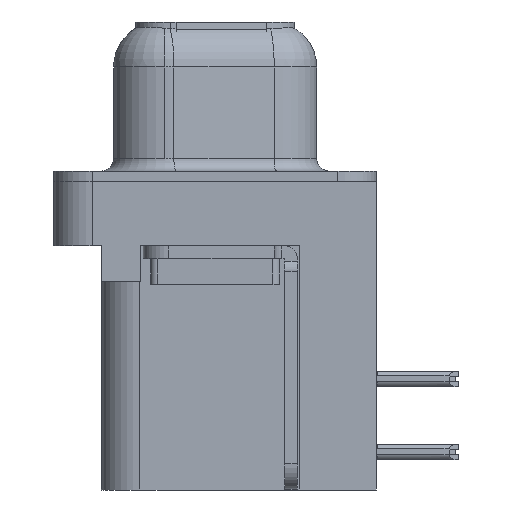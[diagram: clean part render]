
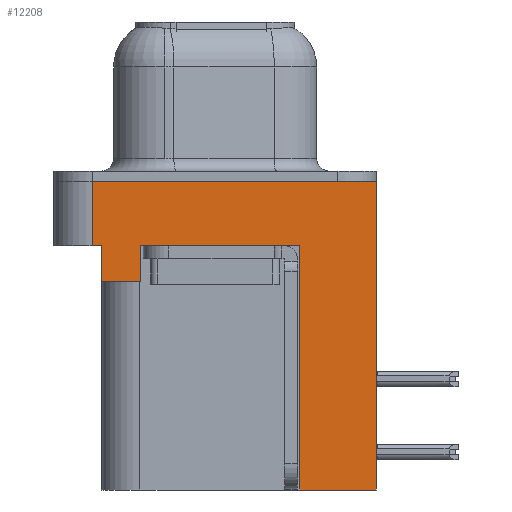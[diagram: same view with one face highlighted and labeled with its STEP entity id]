
A CAD part, left-side view. The second image highlights one B-rep face of the part: STEP entity #12208.
In plain terms, the highlighted planar face has unit normal (-1, 0, 0).
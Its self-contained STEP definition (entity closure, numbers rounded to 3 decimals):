
#340 = CARTESIAN_POINT ( 'NONE',  ( -2.935, -3.295, -12. ) ) ;
#688 = VECTOR ( 'NONE', #11661, 1000. ) ;
#2123 = ORIENTED_EDGE ( 'NONE', *, *, #8368, .T. ) ;
#2290 = VERTEX_POINT ( 'NONE', #4597 ) ;
#2945 = DIRECTION ( 'NONE',  ( 0., 1., 0. ) ) ;
#3043 = VECTOR ( 'NONE', #2945, 1000. ) ;
#3306 = LINE ( 'NONE', #11195, #10658 ) ;
#3784 = DIRECTION ( 'NONE',  ( 0., 0., 1. ) ) ;
#3956 = CARTESIAN_POINT ( 'NONE',  ( -2.935, 4.425, -2.5 ) ) ;
#4115 = CARTESIAN_POINT ( 'NONE',  ( -2.935, -6.275, -12. ) ) ;
#4206 = LINE ( 'NONE', #7159, #24124 ) ;
#4376 = LINE ( 'NONE', #13877, #18670 ) ;
#4496 = DIRECTION ( 'NONE',  ( -1., 0., 0. ) ) ;
#4597 = CARTESIAN_POINT ( 'NONE',  ( -2.935, 2.895, -3.9 ) ) ;
#4629 = VERTEX_POINT ( 'NONE', #3956 ) ;
#6238 = ORIENTED_EDGE ( 'NONE', *, *, #11624, .F. ) ;
#6463 = EDGE_CURVE ( 'NONE', #16593, #17654, #14991, .T. ) ;
#6527 = AXIS2_PLACEMENT_3D ( 'NONE', #8168, #4496, #8004 ) ;
#6555 = EDGE_CURVE ( 'NONE', #14158, #4629, #6859, .T. ) ;
#6666 = VERTEX_POINT ( 'NONE', #22848 ) ;
#6706 = ORIENTED_EDGE ( 'NONE', *, *, #14204, .T. ) ;
#6859 = LINE ( 'NONE', #7821, #688 ) ;
#7085 = VERTEX_POINT ( 'NONE', #7729 ) ;
#7159 = CARTESIAN_POINT ( 'NONE',  ( -2.935, 4.425, -3.9 ) ) ;
#7170 = VERTEX_POINT ( 'NONE', #15617 ) ;
#7499 = LINE ( 'NONE', #19572, #13306 ) ;
#7729 = CARTESIAN_POINT ( 'NONE',  ( -2.935, -6.275, 0. ) ) ;
#7821 = CARTESIAN_POINT ( 'NONE',  ( -2.935, -6.275, -2.5 ) ) ;
#8004 = DIRECTION ( 'NONE',  ( 0., 0., 1. ) ) ;
#8168 = CARTESIAN_POINT ( 'NONE',  ( -2.935, -6.275, -2.5 ) ) ;
#8250 = ORIENTED_EDGE ( 'NONE', *, *, #14344, .F. ) ;
#8368 = EDGE_CURVE ( 'NONE', #16593, #7085, #20469, .T. ) ;
#8672 = EDGE_CURVE ( 'NONE', #18747, #19963, #4376, .T. ) ;
#9219 = CARTESIAN_POINT ( 'NONE',  ( -2.935, -6.275, -2.5 ) ) ;
#9543 = CARTESIAN_POINT ( 'NONE',  ( -2.935, 4.775, -2.5 ) ) ;
#10170 = CARTESIAN_POINT ( 'NONE',  ( -2.935, -3.295, -2.5 ) ) ;
#10252 = EDGE_LOOP ( 'NONE', ( #8250, #13686, #12657, #17006, #13328, #6706, #18015, #6238, #13314, #2123 ) ) ;
#10658 = VECTOR ( 'NONE', #18419, 1000. ) ;
#11195 = CARTESIAN_POINT ( 'NONE',  ( -2.935, -6.275, 0. ) ) ;
#11624 = EDGE_CURVE ( 'NONE', #17654, #19963, #7499, .T. ) ;
#11661 = DIRECTION ( 'NONE',  ( 0., -1., 0. ) ) ;
#11839 = DIRECTION ( 'NONE',  ( 0., 0., 1. ) ) ;
#12208 = ADVANCED_FACE ( 'NONE', ( #16231 ), #19169, .T. ) ;
#12657 = ORIENTED_EDGE ( 'NONE', *, *, #6555, .T. ) ;
#13236 = LINE ( 'NONE', #18061, #14103 ) ;
#13306 = VECTOR ( 'NONE', #13767, 1000. ) ;
#13314 = ORIENTED_EDGE ( 'NONE', *, *, #6463, .F. ) ;
#13328 = ORIENTED_EDGE ( 'NONE', *, *, #15797, .F. ) ;
#13686 = ORIENTED_EDGE ( 'NONE', *, *, #20826, .F. ) ;
#13767 = DIRECTION ( 'NONE',  ( 0., 0., 1. ) ) ;
#13877 = CARTESIAN_POINT ( 'NONE',  ( -2.935, -6.275, -2.5 ) ) ;
#14103 = VECTOR ( 'NONE', #18790, 1000. ) ;
#14113 = CARTESIAN_POINT ( 'NONE',  ( -2.935, -3.295, -12. ) ) ;
#14158 = VERTEX_POINT ( 'NONE', #9543 ) ;
#14204 = EDGE_CURVE ( 'NONE', #2290, #18747, #13236, .T. ) ;
#14344 = EDGE_CURVE ( 'NONE', #6666, #7085, #3306, .T. ) ;
#14991 = LINE ( 'NONE', #14113, #3043 ) ;
#15617 = CARTESIAN_POINT ( 'NONE',  ( -2.935, 4.425, -3.9 ) ) ;
#15797 = EDGE_CURVE ( 'NONE', #2290, #7170, #21325, .T. ) ;
#16101 = CARTESIAN_POINT ( 'NONE',  ( -2.935, 2.895, -2.5 ) ) ;
#16231 = FACE_OUTER_BOUND ( 'NONE', #10252, .T. ) ;
#16593 = VERTEX_POINT ( 'NONE', #4115 ) ;
#16674 = VECTOR ( 'NONE', #3784, 1000. ) ;
#17006 = ORIENTED_EDGE ( 'NONE', *, *, #18472, .F. ) ;
#17228 = DIRECTION ( 'NONE',  ( 0., -1., 0. ) ) ;
#17654 = VERTEX_POINT ( 'NONE', #340 ) ;
#18015 = ORIENTED_EDGE ( 'NONE', *, *, #8672, .T. ) ;
#18061 = CARTESIAN_POINT ( 'NONE',  ( -2.935, 2.895, -3.9 ) ) ;
#18417 = VECTOR ( 'NONE', #11839, 1000. ) ;
#18419 = DIRECTION ( 'NONE',  ( 0., -1., 0. ) ) ;
#18472 = EDGE_CURVE ( 'NONE', #7170, #4629, #4206, .T. ) ;
#18588 = DIRECTION ( 'NONE',  ( 0., 1., 0. ) ) ;
#18670 = VECTOR ( 'NONE', #17228, 1000. ) ;
#18747 = VERTEX_POINT ( 'NONE', #16101 ) ;
#18790 = DIRECTION ( 'NONE',  ( 0., 0., 1. ) ) ;
#18980 = LINE ( 'NONE', #21056, #18417 ) ;
#19169 = PLANE ( 'NONE',  #6527 ) ;
#19572 = CARTESIAN_POINT ( 'NONE',  ( -2.935, -3.295, -12. ) ) ;
#19963 = VERTEX_POINT ( 'NONE', #10170 ) ;
#20469 = LINE ( 'NONE', #9219, #16674 ) ;
#20826 = EDGE_CURVE ( 'NONE', #14158, #6666, #18980, .T. ) ;
#21056 = CARTESIAN_POINT ( 'NONE',  ( -2.935, 4.775, -2.5 ) ) ;
#21325 = LINE ( 'NONE', #22130, #23098 ) ;
#22130 = CARTESIAN_POINT ( 'NONE',  ( -2.935, 4.425, -3.9 ) ) ;
#22848 = CARTESIAN_POINT ( 'NONE',  ( -2.935, 4.775, 0. ) ) ;
#23098 = VECTOR ( 'NONE', #18588, 1000. ) ;
#24066 = DIRECTION ( 'NONE',  ( 0., 0., 1. ) ) ;
#24124 = VECTOR ( 'NONE', #24066, 1000. ) ;
